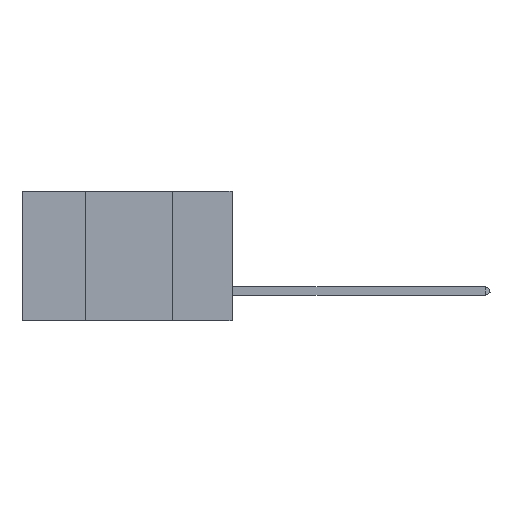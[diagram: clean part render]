
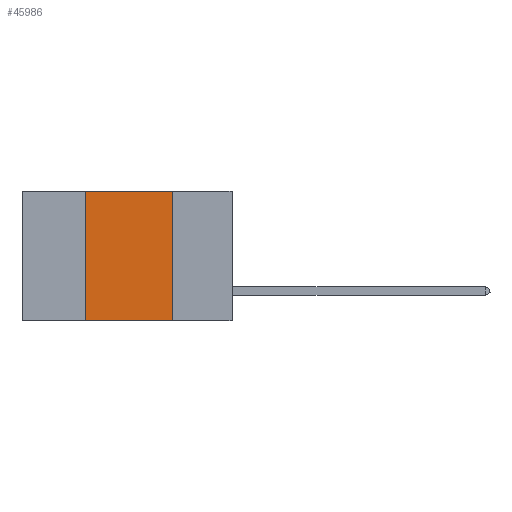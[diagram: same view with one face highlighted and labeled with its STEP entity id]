
A CAD part, left-side view. The second image highlights one B-rep face of the part: STEP entity #45986.
In plain terms, the highlighted planar face has unit normal (-1, 0, 0).
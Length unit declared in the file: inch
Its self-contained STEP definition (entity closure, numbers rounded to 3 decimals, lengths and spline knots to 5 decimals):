
#386 = AXIS2_PLACEMENT_3D ( 'NONE', #14717, #18405, #7652 ) ;
#1117 = CARTESIAN_POINT ( 'NONE',  ( 0., 0.42, -0.37 ) ) ;
#1323 = DIRECTION ( 'NONE',  ( 0., 0., -1. ) ) ;
#2696 = VERTEX_POINT ( 'NONE', #8596 ) ;
#3995 = EDGE_CURVE ( 'NONE', #2696, #44720, #43137, .T. ) ;
#5251 = CARTESIAN_POINT ( 'NONE',  ( 0., 0.6, 0. ) ) ;
#5527 = VERTEX_POINT ( 'NONE', #1117 ) ;
#7652 = DIRECTION ( 'NONE',  ( 0., 0., -1. ) ) ;
#8175 = LINE ( 'NONE', #8210, #19070 ) ;
#8210 = CARTESIAN_POINT ( 'NONE',  ( 0., 0.42, 0. ) ) ;
#8322 = CARTESIAN_POINT ( 'NONE',  ( 0., 0.17, 0. ) ) ;
#8596 = CARTESIAN_POINT ( 'NONE',  ( 0., 0.17, 0. ) ) ;
#8694 = DIRECTION ( 'NONE',  ( 0., 0., 1. ) ) ;
#11333 = PLANE ( 'NONE',  #386 ) ;
#12323 = EDGE_LOOP ( 'NONE', ( #12647, #28575, #31984, #43447 ) ) ;
#12368 = VECTOR ( 'NONE', #1323, 39.37008 ) ;
#12647 = ORIENTED_EDGE ( 'NONE', *, *, #3995, .F. ) ;
#14717 = CARTESIAN_POINT ( 'NONE',  ( 0., 0.6, 0. ) ) ;
#17987 = CARTESIAN_POINT ( 'NONE',  ( 0., 0.6, -0.37 ) ) ;
#18249 = VERTEX_POINT ( 'NONE', #38950 ) ;
#18405 = DIRECTION ( 'NONE',  ( 1., 0., 0. ) ) ;
#19070 = VECTOR ( 'NONE', #8694, 39.37008 ) ;
#20864 = EDGE_CURVE ( 'NONE', #18249, #2696, #28384, .T. ) ;
#23637 = DIRECTION ( 'NONE',  ( 0., -1., 0. ) ) ;
#25066 = EDGE_CURVE ( 'NONE', #5527, #18249, #8175, .T. ) ;
#25278 = LINE ( 'NONE', #17987, #26392 ) ;
#26392 = VECTOR ( 'NONE', #45797, 39.37008 ) ;
#28384 = LINE ( 'NONE', #5251, #35830 ) ;
#28575 = ORIENTED_EDGE ( 'NONE', *, *, #20864, .F. ) ;
#31703 = FACE_OUTER_BOUND ( 'NONE', #12323, .T. ) ;
#31984 = ORIENTED_EDGE ( 'NONE', *, *, #25066, .F. ) ;
#32940 = EDGE_CURVE ( 'NONE', #5527, #44720, #25278, .T. ) ;
#35830 = VECTOR ( 'NONE', #23637, 39.37008 ) ;
#38950 = CARTESIAN_POINT ( 'NONE',  ( 0., 0.42, 0. ) ) ;
#43137 = LINE ( 'NONE', #8322, #12368 ) ;
#43447 = ORIENTED_EDGE ( 'NONE', *, *, #32940, .T. ) ;
#44720 = VERTEX_POINT ( 'NONE', #46202 ) ;
#45797 = DIRECTION ( 'NONE',  ( 0., -1., 0. ) ) ;
#45986 = ADVANCED_FACE ( 'NONE', ( #31703 ), #11333, .F. ) ;
#46202 = CARTESIAN_POINT ( 'NONE',  ( 0., 0.17, -0.37 ) ) ;
